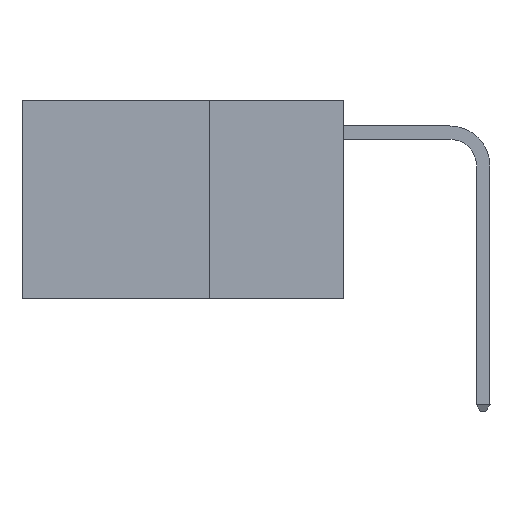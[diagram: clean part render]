
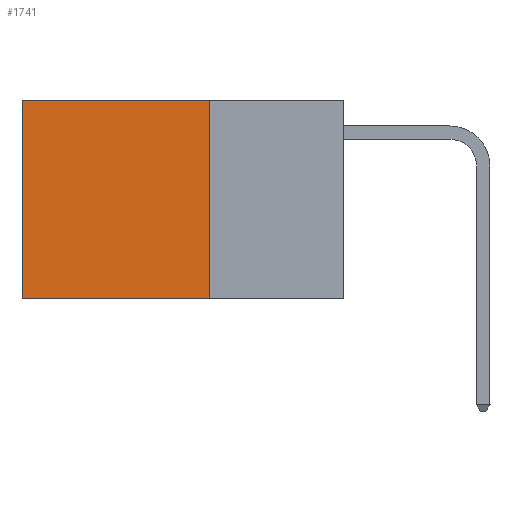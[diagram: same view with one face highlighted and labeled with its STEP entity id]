
A CAD part, left-side view. The second image highlights one B-rep face of the part: STEP entity #1741.
In plain terms, the highlighted planar face has unit normal (-1, 0, 0).
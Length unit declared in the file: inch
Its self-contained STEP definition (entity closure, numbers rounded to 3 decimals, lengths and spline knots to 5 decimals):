
#161 = EDGE_CURVE ( 'NONE', #6295, #11856, #3224, .T. ) ;
#209 = CARTESIAN_POINT ( 'NONE',  ( 0.2625, 0.25, 0. ) ) ;
#576 = LINE ( 'NONE', #209, #11100 ) ;
#869 = DIRECTION ( 'NONE',  ( 0., 0., -1. ) ) ;
#1047 = CARTESIAN_POINT ( 'NONE',  ( 0.2625, 0.6, -0.37 ) ) ;
#1698 = FACE_OUTER_BOUND ( 'NONE', #10074, .T. ) ;
#1741 = ADVANCED_FACE ( 'NONE', ( #1698 ), #8663, .F. ) ;
#1948 = DIRECTION ( 'NONE',  ( 0., 1., 0. ) ) ;
#2118 = CARTESIAN_POINT ( 'NONE',  ( 0.2625, 0.25, 0. ) ) ;
#3083 = VECTOR ( 'NONE', #12087, 39.37008 ) ;
#3224 = LINE ( 'NONE', #4941, #3083 ) ;
#3561 = VECTOR ( 'NONE', #1948, 39.37008 ) ;
#3816 = CARTESIAN_POINT ( 'NONE',  ( 0.2625, 0.25, 0. ) ) ;
#4941 = CARTESIAN_POINT ( 'NONE',  ( 0.2625, 0.25, -0.37 ) ) ;
#5070 = EDGE_CURVE ( 'NONE', #9662, #11856, #8485, .T. ) ;
#5928 = DIRECTION ( 'NONE',  ( 0., 0., -1. ) ) ;
#5948 = VECTOR ( 'NONE', #6181, 39.37008 ) ;
#6181 = DIRECTION ( 'NONE',  ( 0., 0., -1. ) ) ;
#6198 = CARTESIAN_POINT ( 'NONE',  ( 0.2625, 0.6, 0. ) ) ;
#6295 = VERTEX_POINT ( 'NONE', #8600 ) ;
#7252 = CARTESIAN_POINT ( 'NONE',  ( 0.2625, 0.25, 0. ) ) ;
#8485 = LINE ( 'NONE', #6198, #5948 ) ;
#8600 = CARTESIAN_POINT ( 'NONE',  ( 0.2625, 0.25, -0.37 ) ) ;
#8635 = ORIENTED_EDGE ( 'NONE', *, *, #5070, .T. ) ;
#8663 = PLANE ( 'NONE',  #12212 ) ;
#8759 = ORIENTED_EDGE ( 'NONE', *, *, #161, .F. ) ;
#8779 = EDGE_CURVE ( 'NONE', #10964, #6295, #576, .T. ) ;
#8782 = ORIENTED_EDGE ( 'NONE', *, *, #8779, .F. ) ;
#8940 = ORIENTED_EDGE ( 'NONE', *, *, #9991, .T. ) ;
#9662 = VERTEX_POINT ( 'NONE', #11086 ) ;
#9991 = EDGE_CURVE ( 'NONE', #10964, #9662, #10937, .T. ) ;
#10074 = EDGE_LOOP ( 'NONE', ( #8635, #8759, #8782, #8940 ) ) ;
#10572 = DIRECTION ( 'NONE',  ( 1., 0., 0. ) ) ;
#10937 = LINE ( 'NONE', #3816, #3561 ) ;
#10964 = VERTEX_POINT ( 'NONE', #7252 ) ;
#11086 = CARTESIAN_POINT ( 'NONE',  ( 0.2625, 0.6, 0. ) ) ;
#11100 = VECTOR ( 'NONE', #5928, 39.37008 ) ;
#11856 = VERTEX_POINT ( 'NONE', #1047 ) ;
#12087 = DIRECTION ( 'NONE',  ( 0., 1., 0. ) ) ;
#12212 = AXIS2_PLACEMENT_3D ( 'NONE', #2118, #10572, #869 ) ;
